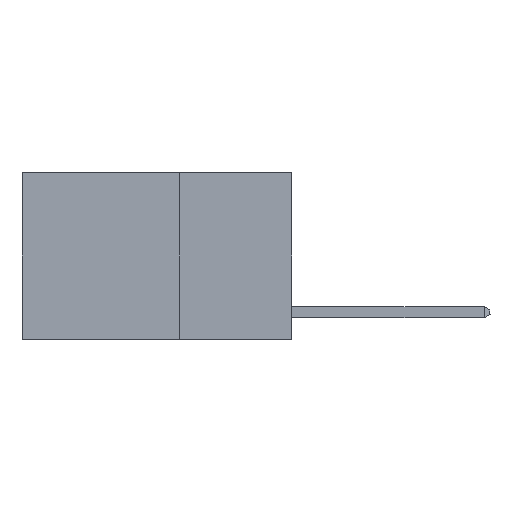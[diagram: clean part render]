
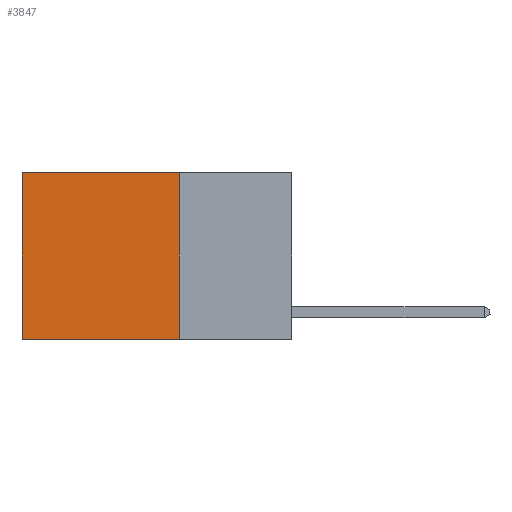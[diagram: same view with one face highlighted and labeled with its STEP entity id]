
A CAD part, left-side view. The second image highlights one B-rep face of the part: STEP entity #3847.
In plain terms, the highlighted planar face has unit normal (-1, 0, 0).
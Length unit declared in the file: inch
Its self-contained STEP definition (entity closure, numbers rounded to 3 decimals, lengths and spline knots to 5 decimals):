
#30 = PLANE ( 'NONE',  #6037 ) ;
#299 = EDGE_CURVE ( 'NONE', #8131, #2650, #13302, .T. ) ;
#302 = VECTOR ( 'NONE', #11814, 39.37008 ) ;
#329 = VERTEX_POINT ( 'NONE', #10182 ) ;
#363 = DIRECTION ( 'NONE',  ( 0., 0., -1. ) ) ;
#431 = LINE ( 'NONE', #7870, #8078 ) ;
#637 = LINE ( 'NONE', #1406, #302 ) ;
#1406 = CARTESIAN_POINT ( 'NONE',  ( 0.2625, 0.25, 0. ) ) ;
#1424 = EDGE_CURVE ( 'NONE', #5145, #2650, #431, .T. ) ;
#1888 = DIRECTION ( 'NONE',  ( 0., 1., 0. ) ) ;
#2142 = DIRECTION ( 'NONE',  ( 1., 0., 0. ) ) ;
#2650 = VERTEX_POINT ( 'NONE', #6322 ) ;
#3267 = CARTESIAN_POINT ( 'NONE',  ( 0.2625, 0.25, -0.37 ) ) ;
#3415 = EDGE_CURVE ( 'NONE', #329, #8131, #637, .T. ) ;
#3772 = EDGE_CURVE ( 'NONE', #329, #5145, #6836, .T. ) ;
#3847 = ADVANCED_FACE ( 'NONE', ( #6198 ), #30, .F. ) ;
#4073 = VECTOR ( 'NONE', #12402, 39.37008 ) ;
#5145 = VERTEX_POINT ( 'NONE', #7291 ) ;
#5165 = CARTESIAN_POINT ( 'NONE',  ( 0.2625, 0.25, 0. ) ) ;
#6037 = AXIS2_PLACEMENT_3D ( 'NONE', #6297, #2142, #9387 ) ;
#6198 = FACE_OUTER_BOUND ( 'NONE', #13179, .T. ) ;
#6297 = CARTESIAN_POINT ( 'NONE',  ( 0.2625, 0.25, 0. ) ) ;
#6322 = CARTESIAN_POINT ( 'NONE',  ( 0.2625, 0.6, -0.37 ) ) ;
#6785 = CARTESIAN_POINT ( 'NONE',  ( 0.2625, 0.25, -0.37 ) ) ;
#6836 = LINE ( 'NONE', #5165, #4073 ) ;
#7190 = ORIENTED_EDGE ( 'NONE', *, *, #3772, .T. ) ;
#7291 = CARTESIAN_POINT ( 'NONE',  ( 0.2625, 0.6, 0. ) ) ;
#7336 = ORIENTED_EDGE ( 'NONE', *, *, #299, .F. ) ;
#7870 = CARTESIAN_POINT ( 'NONE',  ( 0.2625, 0.6, 0. ) ) ;
#8078 = VECTOR ( 'NONE', #363, 39.37008 ) ;
#8131 = VERTEX_POINT ( 'NONE', #6785 ) ;
#8938 = ORIENTED_EDGE ( 'NONE', *, *, #3415, .F. ) ;
#9387 = DIRECTION ( 'NONE',  ( 0., 0., -1. ) ) ;
#10182 = CARTESIAN_POINT ( 'NONE',  ( 0.2625, 0.25, 0. ) ) ;
#10550 = VECTOR ( 'NONE', #1888, 39.37008 ) ;
#11206 = ORIENTED_EDGE ( 'NONE', *, *, #1424, .T. ) ;
#11814 = DIRECTION ( 'NONE',  ( 0., 0., -1. ) ) ;
#12402 = DIRECTION ( 'NONE',  ( 0., 1., 0. ) ) ;
#13179 = EDGE_LOOP ( 'NONE', ( #11206, #7336, #8938, #7190 ) ) ;
#13302 = LINE ( 'NONE', #3267, #10550 ) ;
